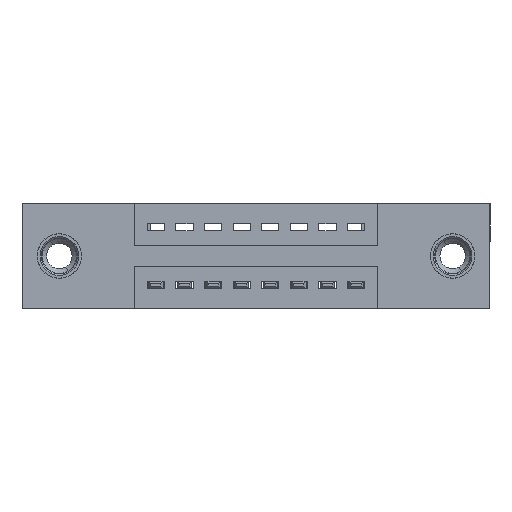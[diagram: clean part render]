
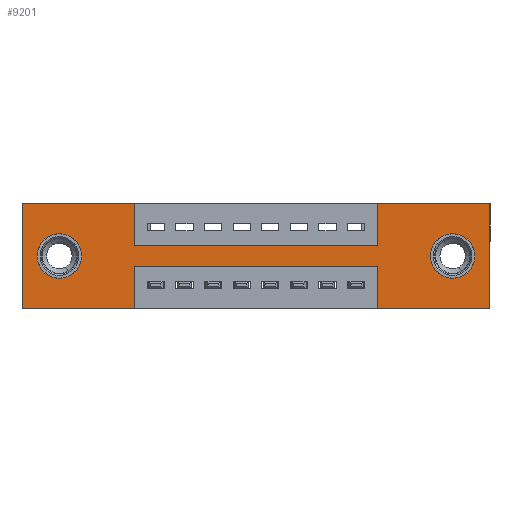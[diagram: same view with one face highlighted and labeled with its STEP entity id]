
A CAD part, front view. The second image highlights one B-rep face of the part: STEP entity #9201.
In plain terms, the highlighted planar face has unit normal (0, -1, 0).
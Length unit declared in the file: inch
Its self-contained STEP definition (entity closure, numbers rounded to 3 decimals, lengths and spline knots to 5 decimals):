
#16 = EDGE_CURVE ( 'NONE', #13318, #4757, #14738, .T. ) ;
#297 = VERTEX_POINT ( 'NONE', #8664 ) ;
#326 = ORIENTED_EDGE ( 'NONE', *, *, #4694, .T. ) ;
#521 = VECTOR ( 'NONE', #6494, 39.37008 ) ;
#551 = AXIS2_PLACEMENT_3D ( 'NONE', #10159, #3024, #3166 ) ;
#937 = CARTESIAN_POINT ( 'NONE',  ( 1.505, 0., -0.185 ) ) ;
#969 = CARTESIAN_POINT ( 'NONE',  ( 1.505, 0., -0.107 ) ) ;
#1133 = DIRECTION ( 'NONE',  ( 0., -1., 0. ) ) ;
#1306 = LINE ( 'NONE', #1500, #10797 ) ;
#1500 = CARTESIAN_POINT ( 'NONE',  ( 0., 0., -0.37 ) ) ;
#1587 = VECTOR ( 'NONE', #4139, 39.37008 ) ;
#1767 = CIRCLE ( 'NONE', #5263, 0.078 ) ;
#1922 = CIRCLE ( 'NONE', #13408, 0.078 ) ;
#2075 = DIRECTION ( 'NONE',  ( 0., 0., -1. ) ) ;
#2145 = CARTESIAN_POINT ( 'NONE',  ( 1.2425, 0., -0.37 ) ) ;
#2148 = VECTOR ( 'NONE', #11107, 39.37008 ) ;
#2308 = ORIENTED_EDGE ( 'NONE', *, *, #6481, .F. ) ;
#2320 = CARTESIAN_POINT ( 'NONE',  ( 1.2425, 0., 0. ) ) ;
#2476 = ORIENTED_EDGE ( 'NONE', *, *, #6561, .F. ) ;
#2805 = DIRECTION ( 'NONE',  ( -1., 0., 0. ) ) ;
#2981 = CARTESIAN_POINT ( 'NONE',  ( 0.3925, 0., -0.37 ) ) ;
#3024 = DIRECTION ( 'NONE',  ( 0., 1., 0. ) ) ;
#3041 = VECTOR ( 'NONE', #7174, 39.37008 ) ;
#3062 = EDGE_CURVE ( 'NONE', #297, #13634, #8551, .T. ) ;
#3162 = ORIENTED_EDGE ( 'NONE', *, *, #4521, .F. ) ;
#3166 = DIRECTION ( 'NONE',  ( 0., 0., 1. ) ) ;
#3276 = VERTEX_POINT ( 'NONE', #13770 ) ;
#3430 = ORIENTED_EDGE ( 'NONE', *, *, #7323, .F. ) ;
#3492 = VERTEX_POINT ( 'NONE', #14731 ) ;
#3658 = DIRECTION ( 'NONE',  ( 0., 0., 1. ) ) ;
#3664 = ORIENTED_EDGE ( 'NONE', *, *, #3062, .F. ) ;
#3750 = CARTESIAN_POINT ( 'NONE',  ( 0.3925, 0., -0.22 ) ) ;
#3799 = DIRECTION ( 'NONE',  ( 0., 1., 0. ) ) ;
#3810 = LINE ( 'NONE', #14088, #12454 ) ;
#3872 = CIRCLE ( 'NONE', #551, 0.078 ) ;
#3891 = VECTOR ( 'NONE', #4265, 39.37008 ) ;
#3896 = EDGE_CURVE ( 'NONE', #6560, #10754, #9368, .T. ) ;
#3929 = ORIENTED_EDGE ( 'NONE', *, *, #4374, .T. ) ;
#4139 = DIRECTION ( 'NONE',  ( -1., 0., 0. ) ) ;
#4154 = LINE ( 'NONE', #12217, #521 ) ;
#4162 = CARTESIAN_POINT ( 'NONE',  ( 0.3925, 0., -0.15 ) ) ;
#4265 = DIRECTION ( 'NONE',  ( 1., 0., 0. ) ) ;
#4374 = EDGE_CURVE ( 'NONE', #11856, #6951, #1922, .T. ) ;
#4521 = EDGE_CURVE ( 'NONE', #6260, #8100, #13070, .T. ) ;
#4540 = LINE ( 'NONE', #4904, #10414 ) ;
#4575 = ORIENTED_EDGE ( 'NONE', *, *, #12442, .F. ) ;
#4669 = FACE_BOUND ( 'NONE', #7793, .T. ) ;
#4694 = EDGE_CURVE ( 'NONE', #6951, #11856, #3872, .T. ) ;
#4757 = VERTEX_POINT ( 'NONE', #969 ) ;
#4904 = CARTESIAN_POINT ( 'NONE',  ( 0.3925, 0., 0. ) ) ;
#4924 = DIRECTION ( 'NONE',  ( 0., 0., 1. ) ) ;
#5027 = EDGE_LOOP ( 'NONE', ( #13650, #3664, #9441, #2308, #2476, #8439, #4575, #13674, #6562, #3162, #3430, #9830 ) ) ;
#5072 = VECTOR ( 'NONE', #2805, 39.37008 ) ;
#5263 = AXIS2_PLACEMENT_3D ( 'NONE', #937, #11660, #2075 ) ;
#5306 = VECTOR ( 'NONE', #11831, 39.37008 ) ;
#5722 = CARTESIAN_POINT ( 'NONE',  ( 0.13, 0., -0.185 ) ) ;
#6035 = CARTESIAN_POINT ( 'NONE',  ( 0., 0., 0. ) ) ;
#6178 = CARTESIAN_POINT ( 'NONE',  ( 0., 0., -0.37 ) ) ;
#6260 = VERTEX_POINT ( 'NONE', #6035 ) ;
#6455 = AXIS2_PLACEMENT_3D ( 'NONE', #11111, #1133, #10174 ) ;
#6481 = EDGE_CURVE ( 'NONE', #3276, #8416, #1306, .T. ) ;
#6490 = CARTESIAN_POINT ( 'NONE',  ( 1.505, 0., -0.185 ) ) ;
#6494 = DIRECTION ( 'NONE',  ( 0., 0., 1. ) ) ;
#6560 = VERTEX_POINT ( 'NONE', #14109 ) ;
#6561 = EDGE_CURVE ( 'NONE', #7400, #3276, #7330, .T. ) ;
#6562 = ORIENTED_EDGE ( 'NONE', *, *, #10853, .F. ) ;
#6684 = DIRECTION ( 'NONE',  ( 0., 0., -1. ) ) ;
#6891 = FACE_OUTER_BOUND ( 'NONE', #5027, .T. ) ;
#6951 = VERTEX_POINT ( 'NONE', #9290 ) ;
#7037 = EDGE_CURVE ( 'NONE', #8416, #297, #12469, .T. ) ;
#7174 = DIRECTION ( 'NONE',  ( 1., 0., 0. ) ) ;
#7189 = EDGE_LOOP ( 'NONE', ( #10554, #13715 ) ) ;
#7323 = EDGE_CURVE ( 'NONE', #14615, #6260, #3810, .T. ) ;
#7330 = LINE ( 'NONE', #14022, #5306 ) ;
#7400 = VERTEX_POINT ( 'NONE', #8570 ) ;
#7507 = CARTESIAN_POINT ( 'NONE',  ( 0., 0., 0. ) ) ;
#7793 = EDGE_LOOP ( 'NONE', ( #3929, #326 ) ) ;
#8100 = VERTEX_POINT ( 'NONE', #9832 ) ;
#8416 = VERTEX_POINT ( 'NONE', #11346 ) ;
#8422 = CARTESIAN_POINT ( 'NONE',  ( 0.3925, 0., -0.22 ) ) ;
#8439 = ORIENTED_EDGE ( 'NONE', *, *, #13651, .F. ) ;
#8551 = LINE ( 'NONE', #3750, #5072 ) ;
#8570 = CARTESIAN_POINT ( 'NONE',  ( 1.635, 0., 0. ) ) ;
#8602 = VECTOR ( 'NONE', #13855, 39.37008 ) ;
#8664 = CARTESIAN_POINT ( 'NONE',  ( 1.2425, 0., -0.22 ) ) ;
#8834 = AXIS2_PLACEMENT_3D ( 'NONE', #6490, #8885, #6684 ) ;
#8885 = DIRECTION ( 'NONE',  ( 0., 1., 0. ) ) ;
#9201 = ADVANCED_FACE ( 'NONE', ( #12760, #4669, #6891 ), #9918, .T. ) ;
#9215 = VERTEX_POINT ( 'NONE', #2320 ) ;
#9290 = CARTESIAN_POINT ( 'NONE',  ( 0.13, 0., -0.263 ) ) ;
#9368 = LINE ( 'NONE', #4162, #3891 ) ;
#9441 = ORIENTED_EDGE ( 'NONE', *, *, #7037, .F. ) ;
#9628 = DIRECTION ( 'NONE',  ( -1., 0., 0. ) ) ;
#9696 = DIRECTION ( 'NONE',  ( 0., 0., -1. ) ) ;
#9738 = EDGE_CURVE ( 'NONE', #3492, #14615, #14774, .T. ) ;
#9781 = EDGE_CURVE ( 'NONE', #13634, #3492, #13676, .T. ) ;
#9830 = ORIENTED_EDGE ( 'NONE', *, *, #9738, .F. ) ;
#9832 = CARTESIAN_POINT ( 'NONE',  ( 0.3925, 0., 0. ) ) ;
#9898 = DIRECTION ( 'NONE',  ( 1., 0., 0. ) ) ;
#9918 = PLANE ( 'NONE',  #6455 ) ;
#10159 = CARTESIAN_POINT ( 'NONE',  ( 0.13, 0., -0.185 ) ) ;
#10174 = DIRECTION ( 'NONE',  ( 0., 0., -1. ) ) ;
#10414 = VECTOR ( 'NONE', #9696, 39.37008 ) ;
#10554 = ORIENTED_EDGE ( 'NONE', *, *, #14061, .T. ) ;
#10754 = VERTEX_POINT ( 'NONE', #11826 ) ;
#10797 = VECTOR ( 'NONE', #9628, 39.37008 ) ;
#10853 = EDGE_CURVE ( 'NONE', #8100, #6560, #4540, .T. ) ;
#11107 = DIRECTION ( 'NONE',  ( 0., 0., -1. ) ) ;
#11111 = CARTESIAN_POINT ( 'NONE',  ( 0., 0., -0.37 ) ) ;
#11258 = LINE ( 'NONE', #14200, #3041 ) ;
#11346 = CARTESIAN_POINT ( 'NONE',  ( 1.2425, 0., -0.37 ) ) ;
#11660 = DIRECTION ( 'NONE',  ( 0., 1., 0. ) ) ;
#11826 = CARTESIAN_POINT ( 'NONE',  ( 1.2425, 0., -0.15 ) ) ;
#11831 = DIRECTION ( 'NONE',  ( 0., 0., -1. ) ) ;
#11856 = VERTEX_POINT ( 'NONE', #13665 ) ;
#12217 = CARTESIAN_POINT ( 'NONE',  ( 1.2425, 0., 0. ) ) ;
#12398 = CARTESIAN_POINT ( 'NONE',  ( 1.505, 0., -0.263 ) ) ;
#12442 = EDGE_CURVE ( 'NONE', #10754, #9215, #4154, .T. ) ;
#12454 = VECTOR ( 'NONE', #3658, 39.37008 ) ;
#12469 = LINE ( 'NONE', #2145, #8602 ) ;
#12515 = CARTESIAN_POINT ( 'NONE',  ( 0., 0., -0.37 ) ) ;
#12699 = VECTOR ( 'NONE', #9898, 39.37008 ) ;
#12760 = FACE_BOUND ( 'NONE', #7189, .T. ) ;
#13070 = LINE ( 'NONE', #7507, #12699 ) ;
#13318 = VERTEX_POINT ( 'NONE', #12398 ) ;
#13408 = AXIS2_PLACEMENT_3D ( 'NONE', #5722, #3799, #4924 ) ;
#13634 = VERTEX_POINT ( 'NONE', #8422 ) ;
#13650 = ORIENTED_EDGE ( 'NONE', *, *, #9781, .F. ) ;
#13651 = EDGE_CURVE ( 'NONE', #9215, #7400, #11258, .T. ) ;
#13665 = CARTESIAN_POINT ( 'NONE',  ( 0.13, 0., -0.107 ) ) ;
#13674 = ORIENTED_EDGE ( 'NONE', *, *, #3896, .F. ) ;
#13676 = LINE ( 'NONE', #2981, #2148 ) ;
#13715 = ORIENTED_EDGE ( 'NONE', *, *, #16, .T. ) ;
#13770 = CARTESIAN_POINT ( 'NONE',  ( 1.635, 0., -0.37 ) ) ;
#13855 = DIRECTION ( 'NONE',  ( 0., 0., 1. ) ) ;
#14022 = CARTESIAN_POINT ( 'NONE',  ( 1.635, 0., 0. ) ) ;
#14061 = EDGE_CURVE ( 'NONE', #4757, #13318, #1767, .T. ) ;
#14088 = CARTESIAN_POINT ( 'NONE',  ( 0., 0., 0. ) ) ;
#14109 = CARTESIAN_POINT ( 'NONE',  ( 0.3925, 0., -0.15 ) ) ;
#14200 = CARTESIAN_POINT ( 'NONE',  ( 0., 0., 0. ) ) ;
#14615 = VERTEX_POINT ( 'NONE', #12515 ) ;
#14731 = CARTESIAN_POINT ( 'NONE',  ( 0.3925, 0., -0.37 ) ) ;
#14738 = CIRCLE ( 'NONE', #8834, 0.078 ) ;
#14774 = LINE ( 'NONE', #6178, #1587 ) ;
